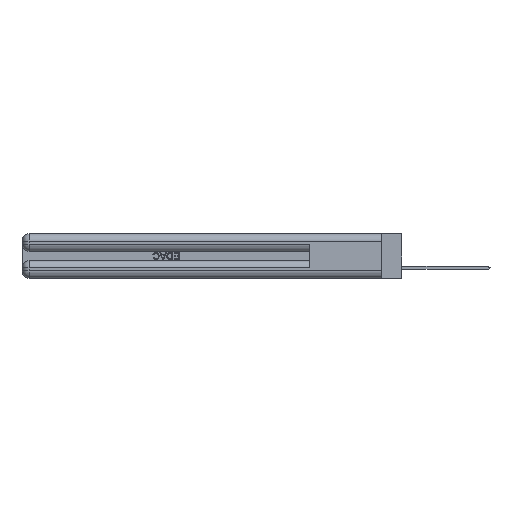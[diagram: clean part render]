
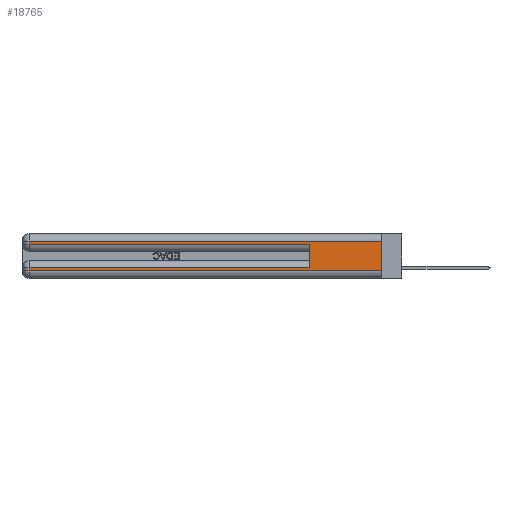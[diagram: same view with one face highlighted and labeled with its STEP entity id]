
A CAD part, left-side view. The second image highlights one B-rep face of the part: STEP entity #18765.
In plain terms, the highlighted planar face has unit normal (-1, 0, 0).
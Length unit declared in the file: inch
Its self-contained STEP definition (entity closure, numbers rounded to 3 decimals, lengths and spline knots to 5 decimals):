
#272 = CARTESIAN_POINT ( 'NONE',  ( 0., 0., 0.31 ) ) ;
#453 = LINE ( 'NONE', #44425, #12610 ) ;
#650 = CARTESIAN_POINT ( 'NONE',  ( 0., 0.6, 0.085 ) ) ;
#1365 = EDGE_CURVE ( 'NONE', #13286, #44132, #31106, .T. ) ;
#2203 = DIRECTION ( 'NONE',  ( 0., 0., -1. ) ) ;
#2397 = PLANE ( 'NONE',  #30875 ) ;
#2549 = DIRECTION ( 'NONE',  ( 1., 0., 0. ) ) ;
#3546 = DIRECTION ( 'NONE',  ( 0., 1., 0. ) ) ;
#4672 = CARTESIAN_POINT ( 'NONE',  ( 0., 2.94, 0.285 ) ) ;
#6332 = CARTESIAN_POINT ( 'NONE',  ( 0., 0., 0.06 ) ) ;
#7093 = ORIENTED_EDGE ( 'NONE', *, *, #39435, .F. ) ;
#7112 = LINE ( 'NONE', #23340, #19258 ) ;
#7629 = VERTEX_POINT ( 'NONE', #4672 ) ;
#8587 = LINE ( 'NONE', #43171, #14699 ) ;
#9107 = ORIENTED_EDGE ( 'NONE', *, *, #26058, .T. ) ;
#12610 = VECTOR ( 'NONE', #34322, 39.37008 ) ;
#12779 = VECTOR ( 'NONE', #33979, 39.37008 ) ;
#13049 = CARTESIAN_POINT ( 'NONE',  ( 0., 2.94, 0.06 ) ) ;
#13286 = VERTEX_POINT ( 'NONE', #272 ) ;
#13578 = LINE ( 'NONE', #19909, #24030 ) ;
#13819 = EDGE_CURVE ( 'NONE', #17141, #42863, #13578, .T. ) ;
#14699 = VECTOR ( 'NONE', #18631, 39.37008 ) ;
#15233 = VERTEX_POINT ( 'NONE', #27975 ) ;
#16231 = VERTEX_POINT ( 'NONE', #33210 ) ;
#16908 = ORIENTED_EDGE ( 'NONE', *, *, #1365, .T. ) ;
#17141 = VERTEX_POINT ( 'NONE', #35556 ) ;
#17333 = FACE_OUTER_BOUND ( 'NONE', #35447, .T. ) ;
#17638 = ORIENTED_EDGE ( 'NONE', *, *, #38070, .T. ) ;
#17661 = EDGE_CURVE ( 'NONE', #13286, #15233, #7112, .T. ) ;
#18631 = DIRECTION ( 'NONE',  ( 0., 0., 1. ) ) ;
#18765 = ADVANCED_FACE ( 'NONE', ( #17333 ), #2397, .F. ) ;
#19258 = VECTOR ( 'NONE', #2203, 39.37008 ) ;
#19671 = ORIENTED_EDGE ( 'NONE', *, *, #17661, .F. ) ;
#19909 = CARTESIAN_POINT ( 'NONE',  ( 0., 2.94, 0.37 ) ) ;
#20159 = CARTESIAN_POINT ( 'NONE',  ( 0., 0., 0.37 ) ) ;
#21010 = CARTESIAN_POINT ( 'NONE',  ( 0., 0., 0.31 ) ) ;
#21788 = VECTOR ( 'NONE', #3546, 39.37008 ) ;
#22510 = VECTOR ( 'NONE', #34621, 39.37008 ) ;
#23340 = CARTESIAN_POINT ( 'NONE',  ( 0., 0., 0.37 ) ) ;
#24030 = VECTOR ( 'NONE', #41404, 39.37008 ) ;
#24062 = EDGE_CURVE ( 'NONE', #44132, #7629, #453, .T. ) ;
#24064 = ORIENTED_EDGE ( 'NONE', *, *, #24062, .T. ) ;
#24152 = DIRECTION ( 'NONE',  ( 0., 0., -1. ) ) ;
#26058 = EDGE_CURVE ( 'NONE', #31868, #17141, #31466, .T. ) ;
#26594 = LINE ( 'NONE', #34915, #29318 ) ;
#27975 = CARTESIAN_POINT ( 'NONE',  ( 0., 0., 0.06 ) ) ;
#28294 = DIRECTION ( 'NONE',  ( 0., -1., 0. ) ) ;
#29318 = VECTOR ( 'NONE', #28294, 39.37008 ) ;
#30874 = CARTESIAN_POINT ( 'NONE',  ( 0., 0., 0.085 ) ) ;
#30875 = AXIS2_PLACEMENT_3D ( 'NONE', #20159, #2549, #24152 ) ;
#31106 = LINE ( 'NONE', #21010, #21788 ) ;
#31466 = LINE ( 'NONE', #30874, #12779 ) ;
#31512 = ORIENTED_EDGE ( 'NONE', *, *, #13819, .T. ) ;
#31518 = CARTESIAN_POINT ( 'NONE',  ( 0., 2.94, 0.31 ) ) ;
#31868 = VERTEX_POINT ( 'NONE', #650 ) ;
#33210 = CARTESIAN_POINT ( 'NONE',  ( 0., 0.6, 0.285 ) ) ;
#33979 = DIRECTION ( 'NONE',  ( 0., 1., 0. ) ) ;
#34322 = DIRECTION ( 'NONE',  ( 0., 0., -1. ) ) ;
#34621 = DIRECTION ( 'NONE',  ( 0., -1., 0. ) ) ;
#34915 = CARTESIAN_POINT ( 'NONE',  ( 0., 0., 0.285 ) ) ;
#35447 = EDGE_LOOP ( 'NONE', ( #19671, #16908, #24064, #44588, #7093, #9107, #31512, #17638 ) ) ;
#35556 = CARTESIAN_POINT ( 'NONE',  ( 0., 2.94, 0.085 ) ) ;
#35926 = EDGE_CURVE ( 'NONE', #7629, #16231, #26594, .T. ) ;
#36765 = LINE ( 'NONE', #6332, #22510 ) ;
#38070 = EDGE_CURVE ( 'NONE', #42863, #15233, #36765, .T. ) ;
#39435 = EDGE_CURVE ( 'NONE', #31868, #16231, #8587, .T. ) ;
#41404 = DIRECTION ( 'NONE',  ( 0., 0., -1. ) ) ;
#42863 = VERTEX_POINT ( 'NONE', #13049 ) ;
#43171 = CARTESIAN_POINT ( 'NONE',  ( 0., 0.6, 0.145 ) ) ;
#44132 = VERTEX_POINT ( 'NONE', #31518 ) ;
#44425 = CARTESIAN_POINT ( 'NONE',  ( 0., 2.94, 0.37 ) ) ;
#44588 = ORIENTED_EDGE ( 'NONE', *, *, #35926, .T. ) ;
